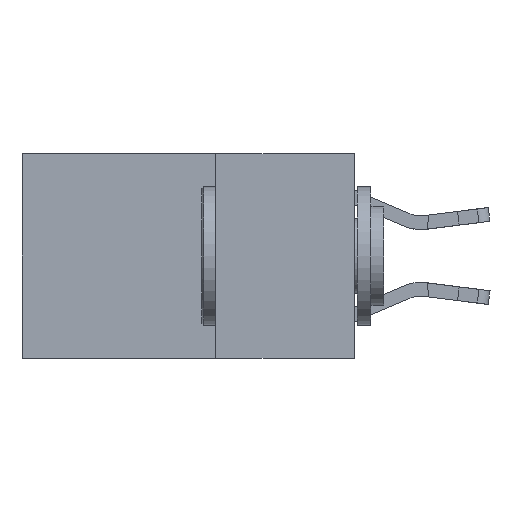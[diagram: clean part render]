
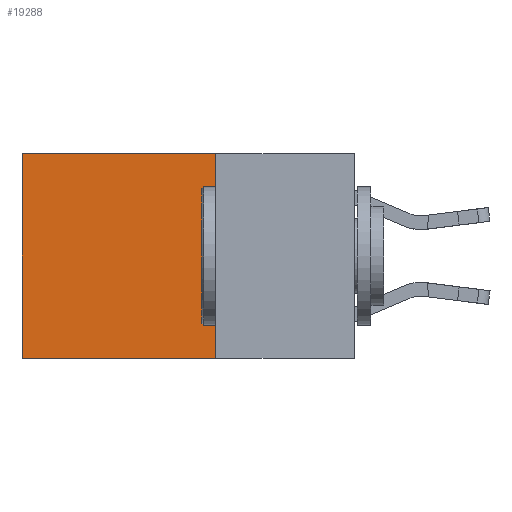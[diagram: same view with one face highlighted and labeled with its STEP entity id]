
A CAD part, left-side view. The second image highlights one B-rep face of the part: STEP entity #19288.
In plain terms, the highlighted planar face has unit normal (-1, 0, 0).
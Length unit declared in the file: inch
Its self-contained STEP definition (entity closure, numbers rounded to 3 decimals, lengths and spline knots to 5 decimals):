
#698 = VECTOR ( 'NONE', #22502, 39.37008 ) ;
#2050 = DIRECTION ( 'NONE',  ( 0., 1., 0. ) ) ;
#2515 = DIRECTION ( 'NONE',  ( 0., 0., -1. ) ) ;
#4060 = LINE ( 'NONE', #22186, #13269 ) ;
#4362 = ORIENTED_EDGE ( 'NONE', *, *, #5441, .F. ) ;
#4680 = ORIENTED_EDGE ( 'NONE', *, *, #11403, .T. ) ;
#4748 = PLANE ( 'NONE',  #5576 ) ;
#5441 = EDGE_CURVE ( 'NONE', #7072, #21184, #4060, .T. ) ;
#5576 = AXIS2_PLACEMENT_3D ( 'NONE', #15716, #6605, #19416 ) ;
#5917 = CARTESIAN_POINT ( 'NONE',  ( 0.2625, 0.25, -0.37 ) ) ;
#6033 = VERTEX_POINT ( 'NONE', #9189 ) ;
#6219 = LINE ( 'NONE', #13419, #698 ) ;
#6605 = DIRECTION ( 'NONE',  ( 1., 0., 0. ) ) ;
#6762 = LINE ( 'NONE', #12600, #15908 ) ;
#7072 = VERTEX_POINT ( 'NONE', #5917 ) ;
#8116 = CARTESIAN_POINT ( 'NONE',  ( 0.2625, 0.6, 0. ) ) ;
#8476 = VECTOR ( 'NONE', #2515, 39.37008 ) ;
#9189 = CARTESIAN_POINT ( 'NONE',  ( 0.2625, 0.6, 0. ) ) ;
#10926 = CARTESIAN_POINT ( 'NONE',  ( 0.2625, 0.25, 0. ) ) ;
#10996 = EDGE_CURVE ( 'NONE', #13446, #7072, #6219, .T. ) ;
#11322 = FACE_OUTER_BOUND ( 'NONE', #22333, .T. ) ;
#11403 = EDGE_CURVE ( 'NONE', #13446, #6033, #6762, .T. ) ;
#11744 = EDGE_CURVE ( 'NONE', #6033, #21184, #13897, .T. ) ;
#12600 = CARTESIAN_POINT ( 'NONE',  ( 0.2625, 0.25, 0. ) ) ;
#13269 = VECTOR ( 'NONE', #2050, 39.37008 ) ;
#13419 = CARTESIAN_POINT ( 'NONE',  ( 0.2625, 0.25, 0. ) ) ;
#13446 = VERTEX_POINT ( 'NONE', #10926 ) ;
#13868 = ORIENTED_EDGE ( 'NONE', *, *, #11744, .T. ) ;
#13897 = LINE ( 'NONE', #8116, #8476 ) ;
#15716 = CARTESIAN_POINT ( 'NONE',  ( 0.2625, 0.25, 0. ) ) ;
#15908 = VECTOR ( 'NONE', #16255, 39.37008 ) ;
#16255 = DIRECTION ( 'NONE',  ( 0., 1., 0. ) ) ;
#19288 = ADVANCED_FACE ( 'NONE', ( #11322 ), #4748, .F. ) ;
#19416 = DIRECTION ( 'NONE',  ( 0., 0., -1. ) ) ;
#21166 = CARTESIAN_POINT ( 'NONE',  ( 0.2625, 0.6, -0.37 ) ) ;
#21184 = VERTEX_POINT ( 'NONE', #21166 ) ;
#21245 = ORIENTED_EDGE ( 'NONE', *, *, #10996, .F. ) ;
#22186 = CARTESIAN_POINT ( 'NONE',  ( 0.2625, 0.25, -0.37 ) ) ;
#22333 = EDGE_LOOP ( 'NONE', ( #13868, #4362, #21245, #4680 ) ) ;
#22502 = DIRECTION ( 'NONE',  ( 0., 0., -1. ) ) ;
